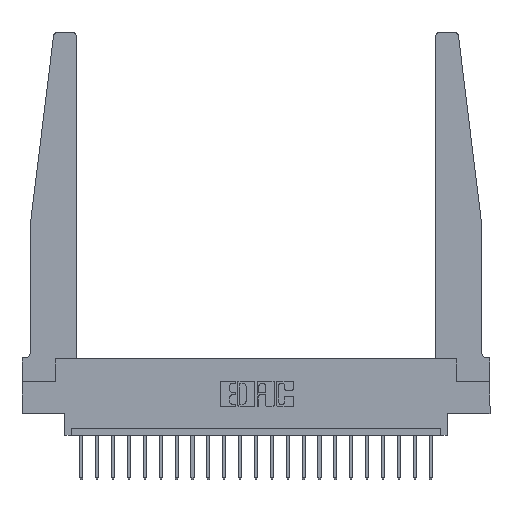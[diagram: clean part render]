
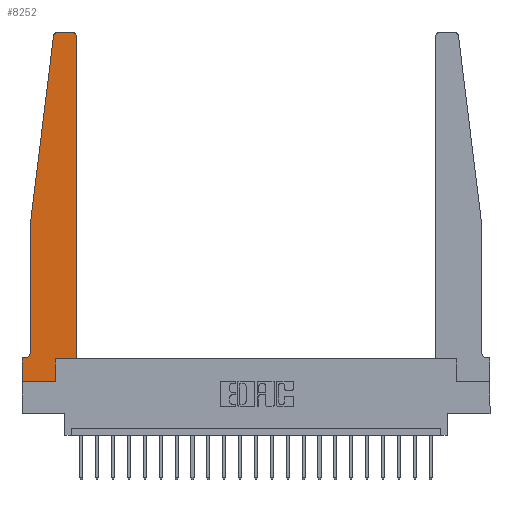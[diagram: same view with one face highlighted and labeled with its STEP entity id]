
A CAD part, top view. The second image highlights one B-rep face of the part: STEP entity #8252.
In plain terms, the highlighted planar face has unit normal (0, 0, 1).
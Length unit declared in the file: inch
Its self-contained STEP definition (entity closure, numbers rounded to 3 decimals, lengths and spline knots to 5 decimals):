
#60 = DIRECTION ( 'NONE',  ( 1., 0., 0. ) ) ;
#177 = EDGE_CURVE ( 'NONE', #16961, #6958, #1453, .T. ) ;
#551 = CARTESIAN_POINT ( 'NONE',  ( 0.27653, 2.72, 0.37 ) ) ;
#605 = LINE ( 'NONE', #9458, #8533 ) ;
#827 = ORIENTED_EDGE ( 'NONE', *, *, #17529, .T. ) ;
#1304 = CARTESIAN_POINT ( 'NONE',  ( 0.24675, 2.72367, 0.37 ) ) ;
#1453 = LINE ( 'NONE', #2501, #18299 ) ;
#1502 = AXIS2_PLACEMENT_3D ( 'NONE', #4798, #21298, #6391 ) ;
#2242 = ORIENTED_EDGE ( 'NONE', *, *, #9646, .T. ) ;
#2311 = ORIENTED_EDGE ( 'NONE', *, *, #177, .T. ) ;
#2499 = FACE_OUTER_BOUND ( 'NONE', #21667, .T. ) ;
#2501 = CARTESIAN_POINT ( 'NONE',  ( 0., 0., 0.37 ) ) ;
#2544 = DIRECTION ( 'NONE',  ( -1., 0., 0. ) ) ;
#2901 = CARTESIAN_POINT ( 'NONE',  ( 0.425, 0.18, 0.37 ) ) ;
#3091 = LINE ( 'NONE', #6610, #17036 ) ;
#3141 = CARTESIAN_POINT ( 'NONE',  ( 0.2605, 0.18, 0.37 ) ) ;
#3310 = VERTEX_POINT ( 'NONE', #12749 ) ;
#3432 = ORIENTED_EDGE ( 'NONE', *, *, #12473, .T. ) ;
#3979 = ORIENTED_EDGE ( 'NONE', *, *, #10527, .T. ) ;
#4157 = VECTOR ( 'NONE', #19579, 39.37008 ) ;
#4334 = CIRCLE ( 'NONE', #15180, 0.03 ) ;
#4378 = CARTESIAN_POINT ( 'NONE',  ( 0.425, 2.72, 0.37 ) ) ;
#4557 = VERTEX_POINT ( 'NONE', #2901 ) ;
#4757 = AXIS2_PLACEMENT_3D ( 'NONE', #17524, #20302, #9354 ) ;
#4798 = CARTESIAN_POINT ( 'NONE',  ( 0.015, 0.2375, 0.37 ) ) ;
#5205 = CARTESIAN_POINT ( 'NONE',  ( 0.065, 0.2375, 0.37 ) ) ;
#5359 = CARTESIAN_POINT ( 'NONE',  ( 0.27653, 2.75, 0.37 ) ) ;
#5427 = DIRECTION ( 'NONE',  ( 0., 1., 0. ) ) ;
#5646 = DIRECTION ( 'NONE',  ( 0., 0., 1. ) ) ;
#5683 = DIRECTION ( 'NONE',  ( 1., 0., 0. ) ) ;
#5948 = ORIENTED_EDGE ( 'NONE', *, *, #6125, .T. ) ;
#6013 = EDGE_CURVE ( 'NONE', #6958, #9074, #9692, .T. ) ;
#6125 = EDGE_CURVE ( 'NONE', #3310, #8441, #21213, .T. ) ;
#6269 = CIRCLE ( 'NONE', #1502, 0.05 ) ;
#6391 = DIRECTION ( 'NONE',  ( -1., 0., 0. ) ) ;
#6418 = CARTESIAN_POINT ( 'NONE',  ( 0.065, 1.25, 0.37 ) ) ;
#6610 = CARTESIAN_POINT ( 'NONE',  ( 0.25, 2.75, 0.37 ) ) ;
#6915 = CARTESIAN_POINT ( 'NONE',  ( 0.015, 0.1875, 0.37 ) ) ;
#6953 = VECTOR ( 'NONE', #16596, 39.37008 ) ;
#6958 = VERTEX_POINT ( 'NONE', #16058 ) ;
#7479 = VERTEX_POINT ( 'NONE', #1304 ) ;
#7861 = VECTOR ( 'NONE', #15840, 39.37008 ) ;
#8252 = ADVANCED_FACE ( 'NONE', ( #2499 ), #15824, .T. ) ;
#8441 = VERTEX_POINT ( 'NONE', #5205 ) ;
#8455 = CARTESIAN_POINT ( 'NONE',  ( 0., 0., 0.37 ) ) ;
#8533 = VECTOR ( 'NONE', #2544, 39.37008 ) ;
#8892 = AXIS2_PLACEMENT_3D ( 'NONE', #20191, #10143, #60 ) ;
#8929 = CARTESIAN_POINT ( 'NONE',  ( 0., 0.1875, 0.37 ) ) ;
#9074 = VERTEX_POINT ( 'NONE', #10326 ) ;
#9183 = CIRCLE ( 'NONE', #8892, 0.03 ) ;
#9354 = DIRECTION ( 'NONE',  ( 1., 0., 0. ) ) ;
#9458 = CARTESIAN_POINT ( 'NONE',  ( 0.065, 0.1875, 0.37 ) ) ;
#9590 = VECTOR ( 'NONE', #5427, 39.37008 ) ;
#9646 = EDGE_CURVE ( 'NONE', #7479, #3310, #12347, .T. ) ;
#9692 = LINE ( 'NONE', #3141, #12574 ) ;
#10143 = DIRECTION ( 'NONE',  ( 0., 0., 1. ) ) ;
#10303 = EDGE_CURVE ( 'NONE', #8441, #12404, #6269, .T. ) ;
#10326 = CARTESIAN_POINT ( 'NONE',  ( 0.2605, 0.18, 0.37 ) ) ;
#10527 = EDGE_CURVE ( 'NONE', #12314, #10688, #3091, .T. ) ;
#10688 = VERTEX_POINT ( 'NONE', #5359 ) ;
#11156 = LINE ( 'NONE', #12122, #9590 ) ;
#11411 = LINE ( 'NONE', #8455, #6953 ) ;
#12117 = CARTESIAN_POINT ( 'NONE',  ( 0.395, 2.75, 0.37 ) ) ;
#12122 = CARTESIAN_POINT ( 'NONE',  ( 0.425, 0.18, 0.37 ) ) ;
#12314 = VERTEX_POINT ( 'NONE', #12117 ) ;
#12347 = LINE ( 'NONE', #6418, #17571 ) ;
#12404 = VERTEX_POINT ( 'NONE', #6915 ) ;
#12473 = EDGE_CURVE ( 'NONE', #10688, #7479, #4334, .T. ) ;
#12512 = EDGE_CURVE ( 'NONE', #4557, #13135, #11156, .T. ) ;
#12574 = VECTOR ( 'NONE', #14874, 39.37008 ) ;
#12749 = CARTESIAN_POINT ( 'NONE',  ( 0.065, 1.25, 0.37 ) ) ;
#13135 = VERTEX_POINT ( 'NONE', #4378 ) ;
#14483 = VERTEX_POINT ( 'NONE', #8929 ) ;
#14507 = ORIENTED_EDGE ( 'NONE', *, *, #12512, .T. ) ;
#14874 = DIRECTION ( 'NONE',  ( 0., 1., 0. ) ) ;
#15119 = ORIENTED_EDGE ( 'NONE', *, *, #17811, .T. ) ;
#15180 = AXIS2_PLACEMENT_3D ( 'NONE', #551, #5646, #15482 ) ;
#15482 = DIRECTION ( 'NONE',  ( 1., 0., 0. ) ) ;
#15824 = PLANE ( 'NONE',  #4757 ) ;
#15840 = DIRECTION ( 'NONE',  ( 1., 0., 0. ) ) ;
#16058 = CARTESIAN_POINT ( 'NONE',  ( 0.2605, 0., 0.37 ) ) ;
#16596 = DIRECTION ( 'NONE',  ( 0., -1., 0. ) ) ;
#16961 = VERTEX_POINT ( 'NONE', #20785 ) ;
#17026 = CARTESIAN_POINT ( 'NONE',  ( 0.065, 1.25, 0.37 ) ) ;
#17036 = VECTOR ( 'NONE', #20261, 39.37008 ) ;
#17524 = CARTESIAN_POINT ( 'NONE',  ( 0., 0.1875, 0.37 ) ) ;
#17529 = EDGE_CURVE ( 'NONE', #14483, #16961, #11411, .T. ) ;
#17571 = VECTOR ( 'NONE', #18195, 39.37008 ) ;
#17811 = EDGE_CURVE ( 'NONE', #12404, #14483, #605, .T. ) ;
#17903 = ORIENTED_EDGE ( 'NONE', *, *, #20512, .T. ) ;
#18195 = DIRECTION ( 'NONE',  ( -0.122, -0.992, 0. ) ) ;
#18299 = VECTOR ( 'NONE', #5683, 39.37008 ) ;
#18566 = ORIENTED_EDGE ( 'NONE', *, *, #6013, .T. ) ;
#18889 = LINE ( 'NONE', #20978, #7861 ) ;
#19147 = ORIENTED_EDGE ( 'NONE', *, *, #10303, .T. ) ;
#19579 = DIRECTION ( 'NONE',  ( 0., -1., 0. ) ) ;
#19586 = ORIENTED_EDGE ( 'NONE', *, *, #20774, .T. ) ;
#20191 = CARTESIAN_POINT ( 'NONE',  ( 0.395, 2.72, 0.37 ) ) ;
#20261 = DIRECTION ( 'NONE',  ( -1., 0., 0. ) ) ;
#20302 = DIRECTION ( 'NONE',  ( 0., 0., 1. ) ) ;
#20512 = EDGE_CURVE ( 'NONE', #13135, #12314, #9183, .T. ) ;
#20774 = EDGE_CURVE ( 'NONE', #9074, #4557, #18889, .T. ) ;
#20785 = CARTESIAN_POINT ( 'NONE',  ( 0., 0., 0.37 ) ) ;
#20978 = CARTESIAN_POINT ( 'NONE',  ( 0.425, 0.18, 0.37 ) ) ;
#21213 = LINE ( 'NONE', #17026, #4157 ) ;
#21298 = DIRECTION ( 'NONE',  ( 0., 0., -1. ) ) ;
#21667 = EDGE_LOOP ( 'NONE', ( #3979, #3432, #2242, #5948, #19147, #15119, #827, #2311, #18566, #19586, #14507, #17903 ) ) ;
